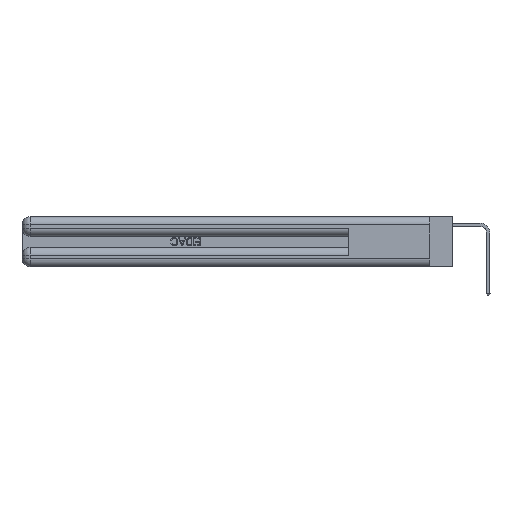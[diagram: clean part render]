
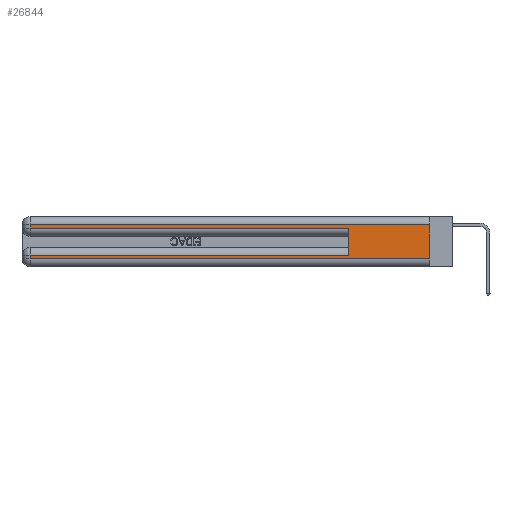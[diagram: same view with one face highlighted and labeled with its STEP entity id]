
A CAD part, left-side view. The second image highlights one B-rep face of the part: STEP entity #26844.
In plain terms, the highlighted planar face has unit normal (-1, 0, 0).
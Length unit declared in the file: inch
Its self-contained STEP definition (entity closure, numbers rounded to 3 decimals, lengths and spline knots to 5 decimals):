
#144 = VECTOR ( 'NONE', #21145, 39.37008 ) ;
#481 = VECTOR ( 'NONE', #11265, 39.37008 ) ;
#731 = ORIENTED_EDGE ( 'NONE', *, *, #30422, .T. ) ;
#1904 = VERTEX_POINT ( 'NONE', #2768 ) ;
#1964 = VECTOR ( 'NONE', #22650, 39.37008 ) ;
#2336 = CARTESIAN_POINT ( 'NONE',  ( 0., 0., 0.06 ) ) ;
#2768 = CARTESIAN_POINT ( 'NONE',  ( 0., 2.94, 0.06 ) ) ;
#3000 = DIRECTION ( 'NONE',  ( 0., 0., -1. ) ) ;
#3255 = PLANE ( 'NONE',  #26733 ) ;
#3430 = VERTEX_POINT ( 'NONE', #28021 ) ;
#3500 = CARTESIAN_POINT ( 'NONE',  ( 0., 2.94, 0.37 ) ) ;
#3678 = EDGE_CURVE ( 'NONE', #3430, #5018, #29798, .T. ) ;
#3948 = CARTESIAN_POINT ( 'NONE',  ( 0., 0., 0.31 ) ) ;
#4913 = LINE ( 'NONE', #10377, #23487 ) ;
#5018 = VERTEX_POINT ( 'NONE', #11661 ) ;
#5834 = DIRECTION ( 'NONE',  ( 0., -1., 0. ) ) ;
#7219 = ORIENTED_EDGE ( 'NONE', *, *, #33185, .F. ) ;
#8727 = CARTESIAN_POINT ( 'NONE',  ( 0., 0., 0.31 ) ) ;
#10377 = CARTESIAN_POINT ( 'NONE',  ( 0., 0., 0.37 ) ) ;
#10534 = VECTOR ( 'NONE', #5834, 39.37008 ) ;
#11133 = VECTOR ( 'NONE', #19038, 39.37008 ) ;
#11265 = DIRECTION ( 'NONE',  ( 0., 1., 0. ) ) ;
#11428 = CARTESIAN_POINT ( 'NONE',  ( 0., 0.6, 0.145 ) ) ;
#11661 = CARTESIAN_POINT ( 'NONE',  ( 0., 2.94, 0.085 ) ) ;
#12835 = CARTESIAN_POINT ( 'NONE',  ( 0., 0.6, 0.285 ) ) ;
#12981 = ORIENTED_EDGE ( 'NONE', *, *, #3678, .T. ) ;
#13104 = ORIENTED_EDGE ( 'NONE', *, *, #26804, .T. ) ;
#13207 = CARTESIAN_POINT ( 'NONE',  ( 0., 2.94, 0.285 ) ) ;
#14009 = CARTESIAN_POINT ( 'NONE',  ( 0., 0., 0.285 ) ) ;
#14420 = EDGE_CURVE ( 'NONE', #29119, #24434, #25036, .T. ) ;
#14435 = VERTEX_POINT ( 'NONE', #34016 ) ;
#14929 = EDGE_CURVE ( 'NONE', #24434, #24519, #28706, .T. ) ;
#16065 = CARTESIAN_POINT ( 'NONE',  ( 0., 0., 0.085 ) ) ;
#17259 = LINE ( 'NONE', #14009, #10534 ) ;
#18984 = CARTESIAN_POINT ( 'NONE',  ( 0., 2.94, 0.31 ) ) ;
#19038 = DIRECTION ( 'NONE',  ( 0., -1., 0. ) ) ;
#19854 = DIRECTION ( 'NONE',  ( 0., 0., -1. ) ) ;
#20168 = ORIENTED_EDGE ( 'NONE', *, *, #25278, .T. ) ;
#20467 = LINE ( 'NONE', #11428, #1964 ) ;
#21136 = VECTOR ( 'NONE', #3000, 39.37008 ) ;
#21145 = DIRECTION ( 'NONE',  ( 0., 1., 0. ) ) ;
#22342 = CARTESIAN_POINT ( 'NONE',  ( 0., 0., 0.37 ) ) ;
#22650 = DIRECTION ( 'NONE',  ( 0., 0., 1. ) ) ;
#23034 = VERTEX_POINT ( 'NONE', #12835 ) ;
#23487 = VECTOR ( 'NONE', #34608, 39.37008 ) ;
#23701 = VECTOR ( 'NONE', #19854, 39.37008 ) ;
#24434 = VERTEX_POINT ( 'NONE', #18984 ) ;
#24519 = VERTEX_POINT ( 'NONE', #13207 ) ;
#25036 = LINE ( 'NONE', #8727, #481 ) ;
#25278 = EDGE_CURVE ( 'NONE', #1904, #14435, #34946, .T. ) ;
#25821 = ORIENTED_EDGE ( 'NONE', *, *, #14420, .T. ) ;
#26733 = AXIS2_PLACEMENT_3D ( 'NONE', #22342, #27935, #33508 ) ;
#26804 = EDGE_CURVE ( 'NONE', #24519, #23034, #17259, .T. ) ;
#26844 = ADVANCED_FACE ( 'NONE', ( #27770 ), #3255, .F. ) ;
#27474 = EDGE_LOOP ( 'NONE', ( #7219, #25821, #28330, #13104, #31268, #12981, #731, #20168 ) ) ;
#27770 = FACE_OUTER_BOUND ( 'NONE', #27474, .T. ) ;
#27857 = CARTESIAN_POINT ( 'NONE',  ( 0., 2.94, 0.37 ) ) ;
#27935 = DIRECTION ( 'NONE',  ( 1., 0., 0. ) ) ;
#28021 = CARTESIAN_POINT ( 'NONE',  ( 0., 0.6, 0.085 ) ) ;
#28330 = ORIENTED_EDGE ( 'NONE', *, *, #14929, .T. ) ;
#28706 = LINE ( 'NONE', #3500, #23701 ) ;
#28976 = EDGE_CURVE ( 'NONE', #3430, #23034, #20467, .T. ) ;
#29119 = VERTEX_POINT ( 'NONE', #3948 ) ;
#29798 = LINE ( 'NONE', #16065, #144 ) ;
#30422 = EDGE_CURVE ( 'NONE', #5018, #1904, #32891, .T. ) ;
#31268 = ORIENTED_EDGE ( 'NONE', *, *, #28976, .F. ) ;
#32891 = LINE ( 'NONE', #27857, #21136 ) ;
#33185 = EDGE_CURVE ( 'NONE', #29119, #14435, #4913, .T. ) ;
#33508 = DIRECTION ( 'NONE',  ( 0., 0., -1. ) ) ;
#34016 = CARTESIAN_POINT ( 'NONE',  ( 0., 0., 0.06 ) ) ;
#34608 = DIRECTION ( 'NONE',  ( 0., 0., -1. ) ) ;
#34946 = LINE ( 'NONE', #2336, #11133 ) ;
